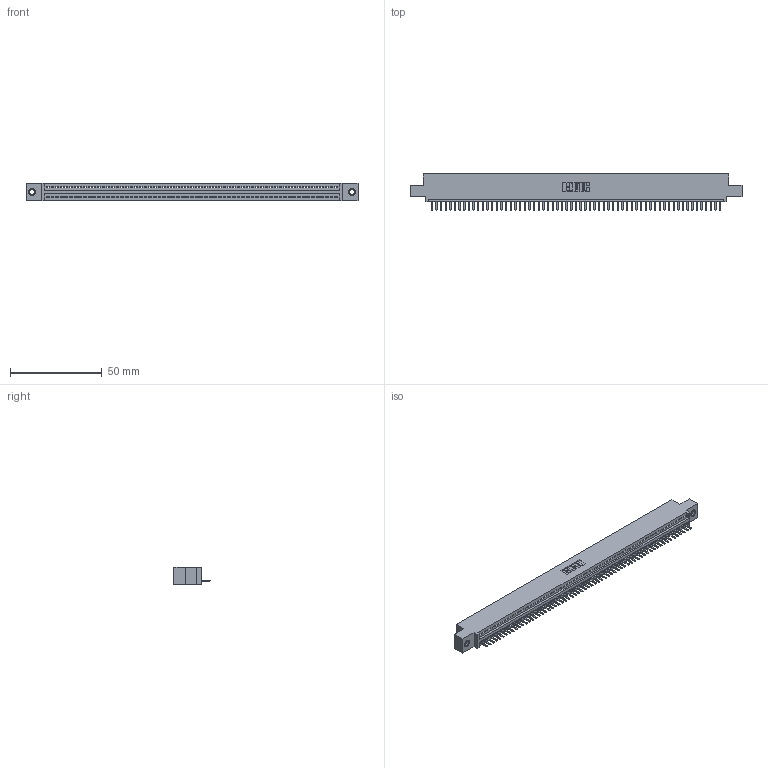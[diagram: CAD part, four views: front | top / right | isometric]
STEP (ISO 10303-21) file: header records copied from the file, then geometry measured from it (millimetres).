
FILE_DESCRIPTION (( 'STEP AP203' ), '1' );
FILE_NAME ('395-063-520-407.STEP', '2019-10-24T20:18:01', ( '' ), ( '' ), 'SwSTEP 2.0', 'SolidWorks 2016', '' );
FILE_SCHEMA (( 'CONFIG_CONTROL_DESIGN' ));
Length unit declared in the file: inch
Products named in the file (4): 395-063-520-407; 345-250-001_345-250-005-103; 345 Part_0.110 Offset - 0.156 Dia-TI; 345-292-001_345-293-120
Assembly tree (66 placements, depth 2):
  395-063-520-407
    345 Part_0.110 Offset - 0.156 Dia-TI
    345-292-001_345-293-120  x63
    345-250-001_345-250-005-103  x2
Bounding box: 181.23 x 19.68 x 9.4 mm (x, y, z)
Volume: 17117.2 mm3; surface area: 22554.3 mm2
Topology: 66 solids, 66 shells, 4096 faces, 12081 edges, 7878 vertices
Faces by surface type: plane 2762, cylinder 1318, cone 12, torus 4
Entity records: 46020 total; most frequent: CARTESIAN_POINT 7964, ORIENTED_EDGE 7942, DIRECTION 6939, EDGE_CURVE 3971, LINE 3563, VECTOR 3563, VERTEX_POINT 2640, AXIS2_PLACEMENT_3D 1688
